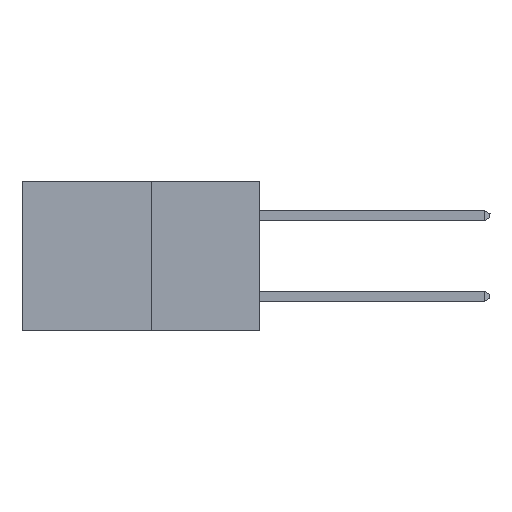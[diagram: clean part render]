
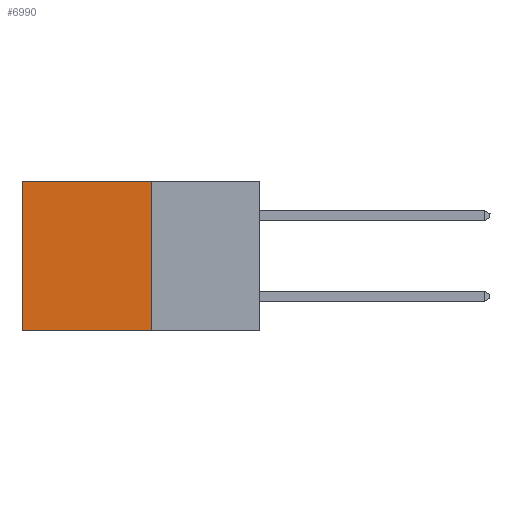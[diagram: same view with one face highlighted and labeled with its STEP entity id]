
A CAD part, left-side view. The second image highlights one B-rep face of the part: STEP entity #6990.
In plain terms, the highlighted planar face has unit normal (-1, 0, 0).
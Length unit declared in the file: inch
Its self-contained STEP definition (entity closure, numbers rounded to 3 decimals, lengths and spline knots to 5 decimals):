
#159 = DIRECTION ( 'NONE',  ( 0., 0., -1. ) ) ;
#203 = EDGE_LOOP ( 'NONE', ( #4263, #7099, #6685, #4462 ) ) ;
#342 = CARTESIAN_POINT ( 'NONE',  ( 0.277, 0.59, -0.37 ) ) ;
#383 = VERTEX_POINT ( 'NONE', #3864 ) ;
#910 = EDGE_CURVE ( 'NONE', #383, #8929, #1312, .T. ) ;
#1312 = LINE ( 'NONE', #342, #8938 ) ;
#2018 = EDGE_CURVE ( 'NONE', #4219, #5042, #2171, .T. ) ;
#2114 = LINE ( 'NONE', #2217, #9187 ) ;
#2171 = LINE ( 'NONE', #6997, #4189 ) ;
#2194 = CARTESIAN_POINT ( 'NONE',  ( 0.277, 0.27, 0. ) ) ;
#2217 = CARTESIAN_POINT ( 'NONE',  ( 0.277, 0.27, -0.37 ) ) ;
#2232 = DIRECTION ( 'NONE',  ( 0., 1., 0. ) ) ;
#2562 = PLANE ( 'NONE',  #4654 ) ;
#3035 = DIRECTION ( 'NONE',  ( 0., 0., -1. ) ) ;
#3176 = FACE_OUTER_BOUND ( 'NONE', #203, .T. ) ;
#3327 = CARTESIAN_POINT ( 'NONE',  ( 0.277, 0.27, -0.37 ) ) ;
#3864 = CARTESIAN_POINT ( 'NONE',  ( 0.277, 0.59, 0. ) ) ;
#4189 = VECTOR ( 'NONE', #5767, 39.37008 ) ;
#4219 = VERTEX_POINT ( 'NONE', #2194 ) ;
#4263 = ORIENTED_EDGE ( 'NONE', *, *, #910, .T. ) ;
#4462 = ORIENTED_EDGE ( 'NONE', *, *, #6757, .T. ) ;
#4654 = AXIS2_PLACEMENT_3D ( 'NONE', #3327, #4873, #159 ) ;
#4873 = DIRECTION ( 'NONE',  ( 1., 0., 0. ) ) ;
#5042 = VERTEX_POINT ( 'NONE', #7930 ) ;
#5182 = CARTESIAN_POINT ( 'NONE',  ( 0.277, 0.27, 0. ) ) ;
#5366 = CARTESIAN_POINT ( 'NONE',  ( 0.277, 0.59, -0.37 ) ) ;
#5369 = EDGE_CURVE ( 'NONE', #5042, #8929, #2114, .T. ) ;
#5767 = DIRECTION ( 'NONE',  ( 0., 0., -1. ) ) ;
#6494 = VECTOR ( 'NONE', #6694, 39.37008 ) ;
#6685 = ORIENTED_EDGE ( 'NONE', *, *, #2018, .F. ) ;
#6694 = DIRECTION ( 'NONE',  ( 0., 1., 0. ) ) ;
#6757 = EDGE_CURVE ( 'NONE', #4219, #383, #7942, .T. ) ;
#6990 = ADVANCED_FACE ( 'NONE', ( #3176 ), #2562, .F. ) ;
#6997 = CARTESIAN_POINT ( 'NONE',  ( 0.277, 0.27, -0.37 ) ) ;
#7099 = ORIENTED_EDGE ( 'NONE', *, *, #5369, .F. ) ;
#7930 = CARTESIAN_POINT ( 'NONE',  ( 0.277, 0.27, -0.37 ) ) ;
#7942 = LINE ( 'NONE', #5182, #6494 ) ;
#8929 = VERTEX_POINT ( 'NONE', #5366 ) ;
#8938 = VECTOR ( 'NONE', #3035, 39.37008 ) ;
#9187 = VECTOR ( 'NONE', #2232, 39.37008 ) ;
